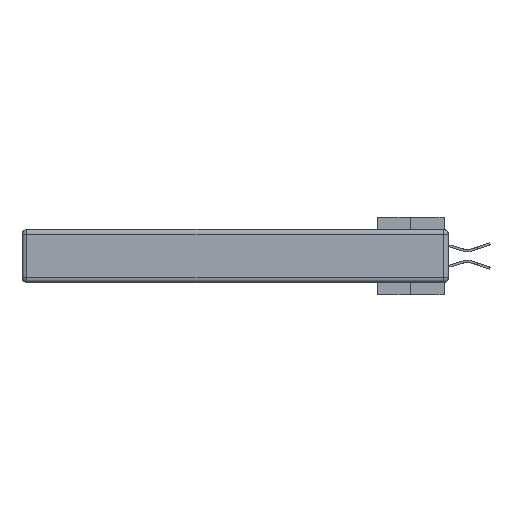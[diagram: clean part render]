
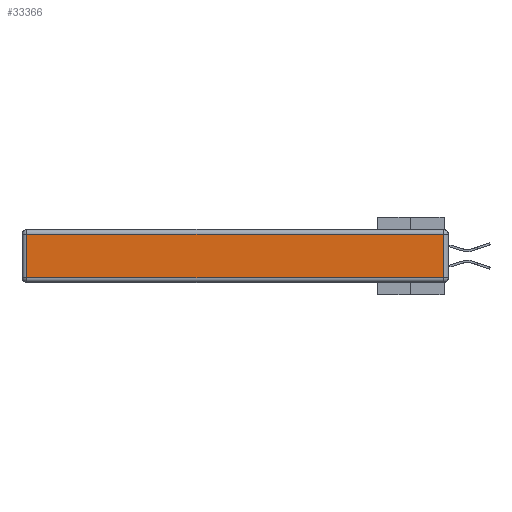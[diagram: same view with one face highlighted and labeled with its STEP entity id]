
A CAD part, left-side view. The second image highlights one B-rep face of the part: STEP entity #33366.
In plain terms, the highlighted planar face has unit normal (-1, 0, 0).
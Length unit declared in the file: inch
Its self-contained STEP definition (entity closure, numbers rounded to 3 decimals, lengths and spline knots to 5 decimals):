
#1268 = ORIENTED_EDGE ( 'NONE', *, *, #27272, .T. ) ;
#2169 = AXIS2_PLACEMENT_3D ( 'NONE', #5583, #43499, #44157 ) ;
#2852 = CARTESIAN_POINT ( 'NONE',  ( 0., 2.75, -0.03 ) ) ;
#4639 = EDGE_LOOP ( 'NONE', ( #39573, #1268, #29886, #39167 ) ) ;
#5232 = PLANE ( 'NONE',  #2169 ) ;
#5406 = CARTESIAN_POINT ( 'NONE',  ( 0., 2.72, -0.03 ) ) ;
#5583 = CARTESIAN_POINT ( 'NONE',  ( 0., 0., -0.343 ) ) ;
#5930 = VECTOR ( 'NONE', #19131, 39.37008 ) ;
#6765 = EDGE_CURVE ( 'NONE', #44803, #48427, #38231, .T. ) ;
#14186 = LINE ( 'NONE', #2852, #34066 ) ;
#14641 = VERTEX_POINT ( 'NONE', #48694 ) ;
#18798 = CARTESIAN_POINT ( 'NONE',  ( 0., 0.03, -0.313 ) ) ;
#18960 = CARTESIAN_POINT ( 'NONE',  ( 0., 2.72, -0.343 ) ) ;
#19131 = DIRECTION ( 'NONE',  ( 0., 0., -1. ) ) ;
#23207 = CARTESIAN_POINT ( 'NONE',  ( 0., 0.03, -0.343 ) ) ;
#26146 = EDGE_CURVE ( 'NONE', #40551, #44803, #42568, .T. ) ;
#26382 = DIRECTION ( 'NONE',  ( 0., 1., 0. ) ) ;
#27221 = DIRECTION ( 'NONE',  ( 0., 0., 1. ) ) ;
#27272 = EDGE_CURVE ( 'NONE', #48427, #14641, #47886, .T. ) ;
#28004 = VECTOR ( 'NONE', #47848, 39.37008 ) ;
#28014 = VECTOR ( 'NONE', #27221, 39.37008 ) ;
#28885 = CARTESIAN_POINT ( 'NONE',  ( 0., 0., -0.313 ) ) ;
#29886 = ORIENTED_EDGE ( 'NONE', *, *, #47799, .T. ) ;
#33366 = ADVANCED_FACE ( 'NONE', ( #49170 ), #5232, .T. ) ;
#34066 = VECTOR ( 'NONE', #26382, 39.37008 ) ;
#36015 = CARTESIAN_POINT ( 'NONE',  ( 0., 2.72, -0.313 ) ) ;
#38231 = LINE ( 'NONE', #28885, #28004 ) ;
#39167 = ORIENTED_EDGE ( 'NONE', *, *, #26146, .T. ) ;
#39573 = ORIENTED_EDGE ( 'NONE', *, *, #6765, .T. ) ;
#40551 = VERTEX_POINT ( 'NONE', #5406 ) ;
#42568 = LINE ( 'NONE', #18960, #5930 ) ;
#43499 = DIRECTION ( 'NONE',  ( -1., 0., 0. ) ) ;
#44157 = DIRECTION ( 'NONE',  ( 0., 0., 1. ) ) ;
#44803 = VERTEX_POINT ( 'NONE', #36015 ) ;
#47799 = EDGE_CURVE ( 'NONE', #14641, #40551, #14186, .T. ) ;
#47848 = DIRECTION ( 'NONE',  ( 0., -1., 0. ) ) ;
#47886 = LINE ( 'NONE', #23207, #28014 ) ;
#48427 = VERTEX_POINT ( 'NONE', #18798 ) ;
#48694 = CARTESIAN_POINT ( 'NONE',  ( 0., 0.03, -0.03 ) ) ;
#49170 = FACE_OUTER_BOUND ( 'NONE', #4639, .T. ) ;
